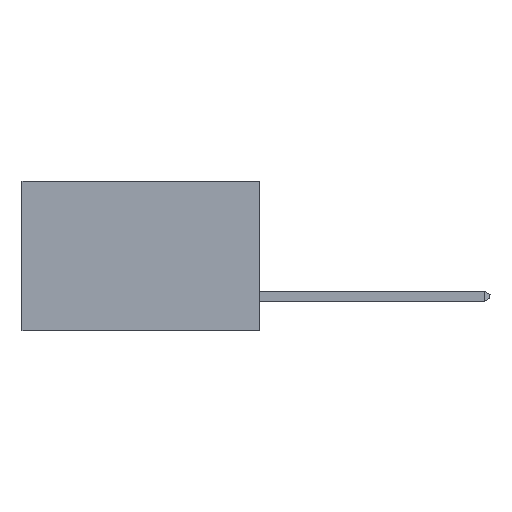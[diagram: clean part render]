
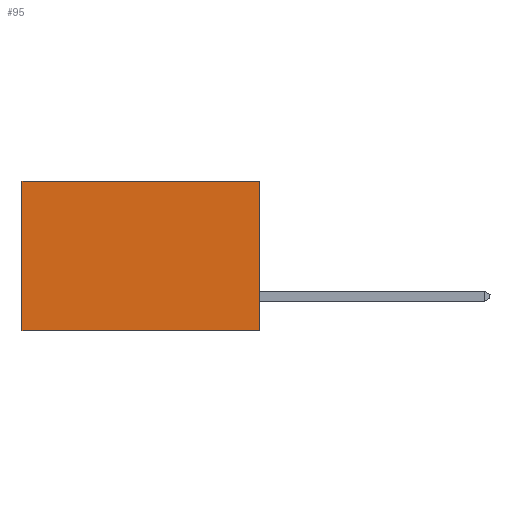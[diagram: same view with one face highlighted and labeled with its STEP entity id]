
A CAD part, left-side view. The second image highlights one B-rep face of the part: STEP entity #95.
In plain terms, the highlighted planar face has unit normal (-1, 0, 0).
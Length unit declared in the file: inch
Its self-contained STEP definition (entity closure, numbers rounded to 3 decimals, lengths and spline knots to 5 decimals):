
#6 = CARTESIAN_POINT ( 'NONE',  ( 0.277, 0., -0.37 ) ) ;
#7 = DIRECTION ( 'NONE',  ( 0., 1., 0. ) ) ;
#95 = ADVANCED_FACE ( 'NONE', ( #1590 ), #2775, .F. ) ;
#355 = EDGE_CURVE ( 'NONE', #917, #5525, #8897, .T. ) ;
#729 = EDGE_LOOP ( 'NONE', ( #5995, #8159, #10126, #6271 ) ) ;
#788 = VECTOR ( 'NONE', #2443, 39.37008 ) ;
#917 = VERTEX_POINT ( 'NONE', #2735 ) ;
#1590 = FACE_OUTER_BOUND ( 'NONE', #729, .T. ) ;
#1619 = VERTEX_POINT ( 'NONE', #9464 ) ;
#2294 = VECTOR ( 'NONE', #7, 39.37008 ) ;
#2443 = DIRECTION ( 'NONE',  ( 0., 1., 0. ) ) ;
#2634 = EDGE_CURVE ( 'NONE', #1619, #917, #9224, .T. ) ;
#2735 = CARTESIAN_POINT ( 'NONE',  ( 0.277, 0.59, 0. ) ) ;
#2775 = PLANE ( 'NONE',  #7708 ) ;
#4490 = DIRECTION ( 'NONE',  ( 0., 0., -1. ) ) ;
#5124 = CARTESIAN_POINT ( 'NONE',  ( 0.277, 0., -0.37 ) ) ;
#5525 = VERTEX_POINT ( 'NONE', #7441 ) ;
#5593 = CARTESIAN_POINT ( 'NONE',  ( 0.277, 0., -0.37 ) ) ;
#5628 = CARTESIAN_POINT ( 'NONE',  ( 0.277, 0., 0. ) ) ;
#5987 = EDGE_CURVE ( 'NONE', #6771, #5525, #6478, .T. ) ;
#5995 = ORIENTED_EDGE ( 'NONE', *, *, #355, .T. ) ;
#6271 = ORIENTED_EDGE ( 'NONE', *, *, #2634, .T. ) ;
#6478 = LINE ( 'NONE', #6, #2294 ) ;
#6771 = VERTEX_POINT ( 'NONE', #10090 ) ;
#7441 = CARTESIAN_POINT ( 'NONE',  ( 0.277, 0.59, -0.37 ) ) ;
#7708 = AXIS2_PLACEMENT_3D ( 'NONE', #5593, #8578, #4490 ) ;
#8090 = CARTESIAN_POINT ( 'NONE',  ( 0.277, 0.59, -0.37 ) ) ;
#8159 = ORIENTED_EDGE ( 'NONE', *, *, #5987, .F. ) ;
#8570 = EDGE_CURVE ( 'NONE', #1619, #6771, #9266, .T. ) ;
#8578 = DIRECTION ( 'NONE',  ( 1., 0., 0. ) ) ;
#8654 = VECTOR ( 'NONE', #9482, 39.37008 ) ;
#8897 = LINE ( 'NONE', #8090, #8654 ) ;
#9030 = VECTOR ( 'NONE', #9112, 39.37008 ) ;
#9112 = DIRECTION ( 'NONE',  ( 0., 0., -1. ) ) ;
#9224 = LINE ( 'NONE', #5628, #788 ) ;
#9266 = LINE ( 'NONE', #5124, #9030 ) ;
#9464 = CARTESIAN_POINT ( 'NONE',  ( 0.277, 0., 0. ) ) ;
#9482 = DIRECTION ( 'NONE',  ( 0., 0., -1. ) ) ;
#10090 = CARTESIAN_POINT ( 'NONE',  ( 0.277, 0., -0.37 ) ) ;
#10126 = ORIENTED_EDGE ( 'NONE', *, *, #8570, .F. ) ;
